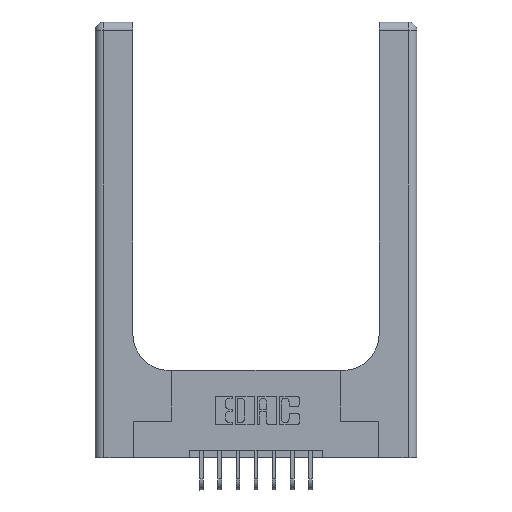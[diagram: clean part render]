
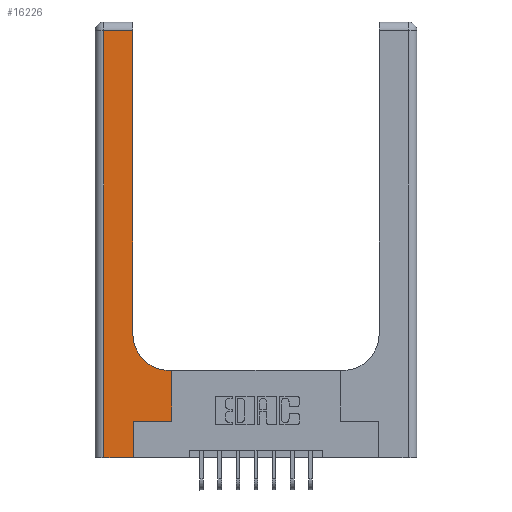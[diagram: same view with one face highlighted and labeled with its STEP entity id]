
A CAD part, top view. The second image highlights one B-rep face of the part: STEP entity #16226.
In plain terms, the highlighted planar face has unit normal (0, 0, 1).
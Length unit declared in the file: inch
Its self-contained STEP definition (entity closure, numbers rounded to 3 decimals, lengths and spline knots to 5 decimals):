
#652 = VERTEX_POINT ( 'NONE', #3306 ) ;
#786 = CARTESIAN_POINT ( 'NONE',  ( 0.06, 2.94, 0.37 ) ) ;
#960 = ORIENTED_EDGE ( 'NONE', *, *, #13407, .T. ) ;
#1479 = LINE ( 'NONE', #3875, #15241 ) ;
#1839 = CARTESIAN_POINT ( 'NONE',  ( 0.06, 0., 0.37 ) ) ;
#1921 = VECTOR ( 'NONE', #5653, 39.37008 ) ;
#2000 = VERTEX_POINT ( 'NONE', #1839 ) ;
#2319 = ORIENTED_EDGE ( 'NONE', *, *, #13813, .T. ) ;
#2409 = CARTESIAN_POINT ( 'NONE',  ( 0.528, 0.6, 0.37 ) ) ;
#3020 = AXIS2_PLACEMENT_3D ( 'NONE', #6089, #11548, #13856 ) ;
#3123 = EDGE_CURVE ( 'NONE', #14282, #8559, #1479, .T. ) ;
#3259 = EDGE_CURVE ( 'NONE', #2000, #10576, #12420, .T. ) ;
#3306 = CARTESIAN_POINT ( 'NONE',  ( 0.51, 0.6, 0.37 ) ) ;
#3392 = LINE ( 'NONE', #9711, #7920 ) ;
#3814 = PLANE ( 'NONE',  #3020 ) ;
#3875 = CARTESIAN_POINT ( 'NONE',  ( 0., 2.94, 0.37 ) ) ;
#3887 = CARTESIAN_POINT ( 'NONE',  ( 0.26, 0.85, 0.37 ) ) ;
#4101 = CARTESIAN_POINT ( 'NONE',  ( 0., 0., 0.37 ) ) ;
#4208 = VECTOR ( 'NONE', #12926, 39.37008 ) ;
#4371 = FACE_OUTER_BOUND ( 'NONE', #12171, .T. ) ;
#4384 = CARTESIAN_POINT ( 'NONE',  ( 0.06, 3., 0.37 ) ) ;
#4406 = VECTOR ( 'NONE', #11707, 39.37008 ) ;
#5653 = DIRECTION ( 'NONE',  ( 0., -1., 0. ) ) ;
#5744 = DIRECTION ( 'NONE',  ( 1., 0., 0. ) ) ;
#5824 = ORIENTED_EDGE ( 'NONE', *, *, #7697, .T. ) ;
#5902 = CIRCLE ( 'NONE', #8998, 0.25 ) ;
#5997 = VECTOR ( 'NONE', #5744, 39.37008 ) ;
#6089 = CARTESIAN_POINT ( 'NONE',  ( 0., 3., 0.37 ) ) ;
#6209 = ORIENTED_EDGE ( 'NONE', *, *, #13840, .T. ) ;
#6415 = EDGE_CURVE ( 'NONE', #15923, #14568, #11610, .T. ) ;
#6582 = VECTOR ( 'NONE', #9078, 39.37008 ) ;
#7160 = ORIENTED_EDGE ( 'NONE', *, *, #15838, .T. ) ;
#7319 = VECTOR ( 'NONE', #12856, 39.37008 ) ;
#7646 = CARTESIAN_POINT ( 'NONE',  ( 0.51, 0.85, 0.37 ) ) ;
#7697 = EDGE_CURVE ( 'NONE', #10576, #15923, #14785, .T. ) ;
#7920 = VECTOR ( 'NONE', #10811, 39.37008 ) ;
#8018 = CARTESIAN_POINT ( 'NONE',  ( 0.528, 0.25, 0.37 ) ) ;
#8119 = LINE ( 'NONE', #8018, #4406 ) ;
#8559 = VERTEX_POINT ( 'NONE', #786 ) ;
#8924 = DIRECTION ( 'NONE',  ( 0., 0., -1. ) ) ;
#8998 = AXIS2_PLACEMENT_3D ( 'NONE', #7646, #8924, #13921 ) ;
#9064 = CARTESIAN_POINT ( 'NONE',  ( 0.265, 0., 0.37 ) ) ;
#9078 = DIRECTION ( 'NONE',  ( 1., 0., 0. ) ) ;
#9548 = VERTEX_POINT ( 'NONE', #2409 ) ;
#9711 = CARTESIAN_POINT ( 'NONE',  ( 0.26, 3., 0.37 ) ) ;
#9798 = ORIENTED_EDGE ( 'NONE', *, *, #3123, .T. ) ;
#10006 = LINE ( 'NONE', #4384, #1921 ) ;
#10576 = VERTEX_POINT ( 'NONE', #9064 ) ;
#10811 = DIRECTION ( 'NONE',  ( 0., 1., 0. ) ) ;
#10830 = EDGE_CURVE ( 'NONE', #14568, #9548, #8119, .T. ) ;
#11548 = DIRECTION ( 'NONE',  ( 0., 0., -1. ) ) ;
#11610 = LINE ( 'NONE', #15759, #5997 ) ;
#11707 = DIRECTION ( 'NONE',  ( 0., 1., 0. ) ) ;
#11713 = CARTESIAN_POINT ( 'NONE',  ( 0.265, 0., 0.37 ) ) ;
#12148 = VERTEX_POINT ( 'NONE', #3887 ) ;
#12171 = EDGE_LOOP ( 'NONE', ( #7160, #9798, #6209, #14613, #5824, #13794, #15881, #2319, #960 ) ) ;
#12420 = LINE ( 'NONE', #4101, #6582 ) ;
#12856 = DIRECTION ( 'NONE',  ( 0., 1., 0. ) ) ;
#12926 = DIRECTION ( 'NONE',  ( -1., 0., 0. ) ) ;
#13407 = EDGE_CURVE ( 'NONE', #652, #12148, #5902, .T. ) ;
#13794 = ORIENTED_EDGE ( 'NONE', *, *, #6415, .T. ) ;
#13813 = EDGE_CURVE ( 'NONE', #9548, #652, #15373, .T. ) ;
#13840 = EDGE_CURVE ( 'NONE', #8559, #2000, #10006, .T. ) ;
#13856 = DIRECTION ( 'NONE',  ( -1., 0., 0. ) ) ;
#13921 = DIRECTION ( 'NONE',  ( 1., 0., 0. ) ) ;
#13942 = CARTESIAN_POINT ( 'NONE',  ( 0.528, 0.25, 0.37 ) ) ;
#14118 = CARTESIAN_POINT ( 'NONE',  ( 0.26, 2.94, 0.37 ) ) ;
#14282 = VERTEX_POINT ( 'NONE', #14118 ) ;
#14568 = VERTEX_POINT ( 'NONE', #13942 ) ;
#14613 = ORIENTED_EDGE ( 'NONE', *, *, #3259, .T. ) ;
#14785 = LINE ( 'NONE', #11713, #7319 ) ;
#15050 = DIRECTION ( 'NONE',  ( -1., 0., 0. ) ) ;
#15241 = VECTOR ( 'NONE', #15050, 39.37008 ) ;
#15373 = LINE ( 'NONE', #15536, #4208 ) ;
#15536 = CARTESIAN_POINT ( 'NONE',  ( 0.26, 0.6, 0.37 ) ) ;
#15759 = CARTESIAN_POINT ( 'NONE',  ( 0.265, 0.25, 0.37 ) ) ;
#15838 = EDGE_CURVE ( 'NONE', #12148, #14282, #3392, .T. ) ;
#15881 = ORIENTED_EDGE ( 'NONE', *, *, #10830, .T. ) ;
#15923 = VERTEX_POINT ( 'NONE', #15934 ) ;
#15934 = CARTESIAN_POINT ( 'NONE',  ( 0.265, 0.25, 0.37 ) ) ;
#16226 = ADVANCED_FACE ( 'NONE', ( #4371 ), #3814, .F. ) ;
